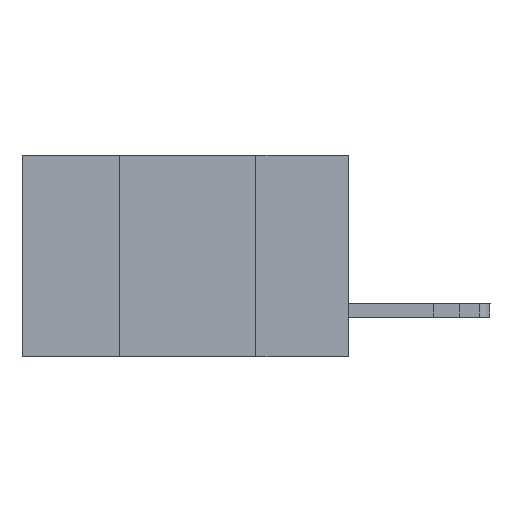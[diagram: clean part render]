
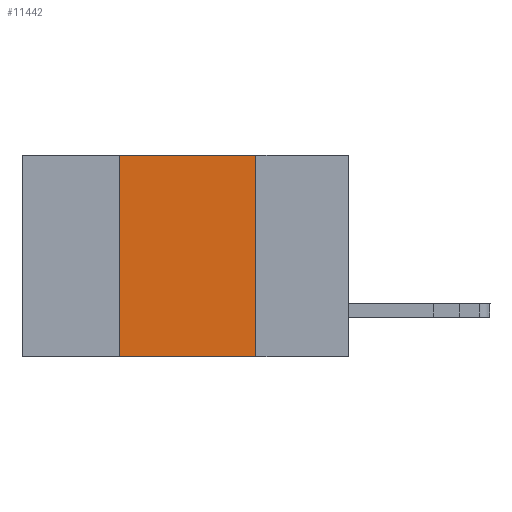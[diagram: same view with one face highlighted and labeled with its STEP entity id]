
A CAD part, left-side view. The second image highlights one B-rep face of the part: STEP entity #11442.
In plain terms, the highlighted planar face has unit normal (-1, 0, 0).
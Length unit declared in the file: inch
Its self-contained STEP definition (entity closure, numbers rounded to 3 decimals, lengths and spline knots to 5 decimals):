
#630 = LINE ( 'NONE', #20126, #10239 ) ;
#971 = VERTEX_POINT ( 'NONE', #9002 ) ;
#1122 = EDGE_CURVE ( 'NONE', #11159, #8843, #14171, .T. ) ;
#2697 = DIRECTION ( 'NONE',  ( 1., 0., 0. ) ) ;
#3967 = DIRECTION ( 'NONE',  ( 0., 0., 1. ) ) ;
#4390 = DIRECTION ( 'NONE',  ( 0., 0., -1. ) ) ;
#4487 = ORIENTED_EDGE ( 'NONE', *, *, #10637, .F. ) ;
#5093 = ORIENTED_EDGE ( 'NONE', *, *, #1122, .T. ) ;
#5948 = DIRECTION ( 'NONE',  ( 0., -1., 0. ) ) ;
#6029 = CARTESIAN_POINT ( 'NONE',  ( 0., 0.17, -0.37 ) ) ;
#6670 = AXIS2_PLACEMENT_3D ( 'NONE', #18705, #2697, #7573 ) ;
#6948 = DIRECTION ( 'NONE',  ( 0., -1., 0. ) ) ;
#7573 = DIRECTION ( 'NONE',  ( 0., 0., -1. ) ) ;
#8054 = VERTEX_POINT ( 'NONE', #14774 ) ;
#8843 = VERTEX_POINT ( 'NONE', #16511 ) ;
#9002 = CARTESIAN_POINT ( 'NONE',  ( 0., 0.17, 0. ) ) ;
#10239 = VECTOR ( 'NONE', #6948, 39.37008 ) ;
#10637 = EDGE_CURVE ( 'NONE', #971, #8843, #17794, .T. ) ;
#10829 = VECTOR ( 'NONE', #4390, 39.37008 ) ;
#11159 = VERTEX_POINT ( 'NONE', #21095 ) ;
#11442 = ADVANCED_FACE ( 'NONE', ( #13953 ), #12461, .F. ) ;
#12461 = PLANE ( 'NONE',  #6670 ) ;
#12980 = VECTOR ( 'NONE', #3967, 39.37008 ) ;
#13545 = EDGE_CURVE ( 'NONE', #11159, #8054, #20382, .T. ) ;
#13953 = FACE_OUTER_BOUND ( 'NONE', #15538, .T. ) ;
#14171 = LINE ( 'NONE', #20742, #20490 ) ;
#14313 = EDGE_CURVE ( 'NONE', #8054, #971, #630, .T. ) ;
#14774 = CARTESIAN_POINT ( 'NONE',  ( 0., 0.42, 0. ) ) ;
#15227 = ORIENTED_EDGE ( 'NONE', *, *, #14313, .F. ) ;
#15538 = EDGE_LOOP ( 'NONE', ( #4487, #15227, #20995, #5093 ) ) ;
#16511 = CARTESIAN_POINT ( 'NONE',  ( 0., 0.17, -0.37 ) ) ;
#17794 = LINE ( 'NONE', #6029, #10829 ) ;
#18705 = CARTESIAN_POINT ( 'NONE',  ( 0., 0.6, 0. ) ) ;
#18761 = CARTESIAN_POINT ( 'NONE',  ( 0., 0.42, -0.37 ) ) ;
#20126 = CARTESIAN_POINT ( 'NONE',  ( 0., 0.6, 0. ) ) ;
#20382 = LINE ( 'NONE', #18761, #12980 ) ;
#20490 = VECTOR ( 'NONE', #5948, 39.37008 ) ;
#20742 = CARTESIAN_POINT ( 'NONE',  ( 0., 0.6, -0.37 ) ) ;
#20995 = ORIENTED_EDGE ( 'NONE', *, *, #13545, .F. ) ;
#21095 = CARTESIAN_POINT ( 'NONE',  ( 0., 0.42, -0.37 ) ) ;
